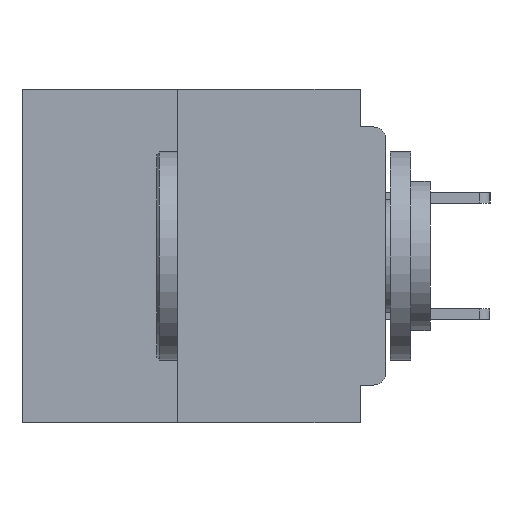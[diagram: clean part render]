
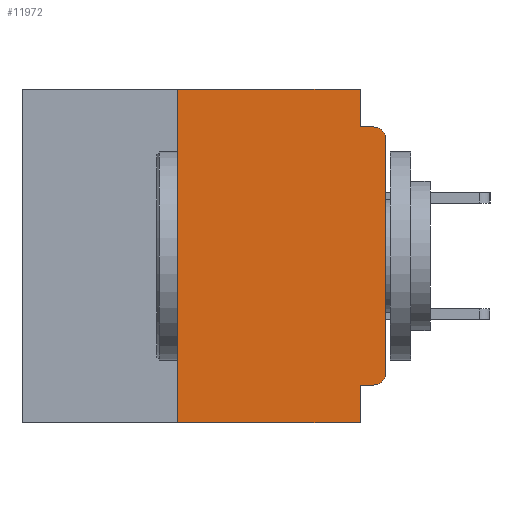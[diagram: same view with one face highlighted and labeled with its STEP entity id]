
A CAD part, left-side view. The second image highlights one B-rep face of the part: STEP entity #11972.
In plain terms, the highlighted planar face has unit normal (-1, 0, 0).
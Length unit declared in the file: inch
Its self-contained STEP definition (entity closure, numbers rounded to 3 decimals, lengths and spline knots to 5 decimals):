
#702 = VERTEX_POINT ( 'NONE', #54843 ) ;
#1811 = VERTEX_POINT ( 'NONE', #20018 ) ;
#4712 = CARTESIAN_POINT ( 'NONE',  ( 0., 0.437, 0. ) ) ;
#7472 = CARTESIAN_POINT ( 'NONE',  ( 0., 0.437, -0.4 ) ) ;
#7946 = EDGE_CURVE ( 'NONE', #57414, #702, #52323, .T. ) ;
#8052 = CARTESIAN_POINT ( 'NONE',  ( 0., 0.031, -0.355 ) ) ;
#8495 = CARTESIAN_POINT ( 'NONE',  ( 0., 0.031, 0. ) ) ;
#9352 = CARTESIAN_POINT ( 'NONE',  ( 0., 0.031, -0.4 ) ) ;
#9737 = VECTOR ( 'NONE', #40722, 39.37008 ) ;
#9796 = DIRECTION ( 'NONE',  ( 0., 1., 0. ) ) ;
#10257 = VERTEX_POINT ( 'NONE', #26224 ) ;
#11354 = LINE ( 'NONE', #14819, #9737 ) ;
#11581 = VECTOR ( 'NONE', #56571, 39.37008 ) ;
#11972 = ADVANCED_FACE ( 'NONE', ( #33590 ), #56384, .F. ) ;
#12123 = CARTESIAN_POINT ( 'NONE',  ( 0., 0.25, 0. ) ) ;
#12883 = CARTESIAN_POINT ( 'NONE',  ( 0., 0.25, -0.4 ) ) ;
#13682 = DIRECTION ( 'NONE',  ( 0., 0., -1. ) ) ;
#14777 = CARTESIAN_POINT ( 'NONE',  ( 0., 0., -0.355 ) ) ;
#14819 = CARTESIAN_POINT ( 'NONE',  ( 0., 0.437, 0. ) ) ;
#15334 = VECTOR ( 'NONE', #64381, 39.37008 ) ;
#15539 = EDGE_CURVE ( 'NONE', #24366, #20336, #37382, .T. ) ;
#15829 = VERTEX_POINT ( 'NONE', #12123 ) ;
#15956 = EDGE_CURVE ( 'NONE', #702, #58829, #66434, .T. ) ;
#17506 = ORIENTED_EDGE ( 'NONE', *, *, #32362, .T. ) ;
#18109 = DIRECTION ( 'NONE',  ( 0., 0., 1. ) ) ;
#18802 = VECTOR ( 'NONE', #18109, 39.37008 ) ;
#20018 = CARTESIAN_POINT ( 'NONE',  ( 0., 0.015, -0.355 ) ) ;
#20336 = VERTEX_POINT ( 'NONE', #33363 ) ;
#20462 = AXIS2_PLACEMENT_3D ( 'NONE', #58294, #27416, #63546 ) ;
#20517 = CARTESIAN_POINT ( 'NONE',  ( 0., 0., 0. ) ) ;
#20711 = ORIENTED_EDGE ( 'NONE', *, *, #48529, .F. ) ;
#21270 = VERTEX_POINT ( 'NONE', #9352 ) ;
#23662 = VECTOR ( 'NONE', #55121, 39.37008 ) ;
#24366 = VERTEX_POINT ( 'NONE', #45286 ) ;
#24946 = VECTOR ( 'NONE', #13682, 39.37008 ) ;
#25868 = DIRECTION ( 'NONE',  ( 0., 0., -1. ) ) ;
#26224 = CARTESIAN_POINT ( 'NONE',  ( 0., 0.25, -0.4 ) ) ;
#27063 = LINE ( 'NONE', #14777, #39095 ) ;
#27416 = DIRECTION ( 'NONE',  ( -1., 0., 0. ) ) ;
#27942 = ORIENTED_EDGE ( 'NONE', *, *, #15539, .T. ) ;
#28408 = EDGE_LOOP ( 'NONE', ( #27942, #17506, #58764, #44585, #45764, #40111, #41410, #20711, #46842, #46403 ) ) ;
#30639 = DIRECTION ( 'NONE',  ( -1., 0., 0. ) ) ;
#30701 = DIRECTION ( 'NONE',  ( 0., 0., -1. ) ) ;
#30741 = VECTOR ( 'NONE', #25868, 39.37008 ) ;
#32362 = EDGE_CURVE ( 'NONE', #20336, #58829, #54423, .T. ) ;
#33363 = CARTESIAN_POINT ( 'NONE',  ( 0., 0., -0.06 ) ) ;
#33590 = FACE_OUTER_BOUND ( 'NONE', #28408, .T. ) ;
#34231 = CIRCLE ( 'NONE', #20462, 0.015 ) ;
#37382 = LINE ( 'NONE', #20517, #11581 ) ;
#37975 = EDGE_CURVE ( 'NONE', #10257, #15829, #44560, .T. ) ;
#38454 = CARTESIAN_POINT ( 'NONE',  ( 0., 0.031, 0. ) ) ;
#39095 = VECTOR ( 'NONE', #9796, 39.37008 ) ;
#40111 = ORIENTED_EDGE ( 'NONE', *, *, #37975, .F. ) ;
#40722 = DIRECTION ( 'NONE',  ( 0., -1., 0. ) ) ;
#40737 = EDGE_CURVE ( 'NONE', #10257, #21270, #56467, .T. ) ;
#41410 = ORIENTED_EDGE ( 'NONE', *, *, #40737, .T. ) ;
#41702 = AXIS2_PLACEMENT_3D ( 'NONE', #4712, #61636, #30701 ) ;
#44442 = LINE ( 'NONE', #56715, #30741 ) ;
#44560 = LINE ( 'NONE', #12883, #18802 ) ;
#44579 = VERTEX_POINT ( 'NONE', #8052 ) ;
#44585 = ORIENTED_EDGE ( 'NONE', *, *, #7946, .F. ) ;
#45286 = CARTESIAN_POINT ( 'NONE',  ( 0., 0., -0.34 ) ) ;
#45764 = ORIENTED_EDGE ( 'NONE', *, *, #54713, .F. ) ;
#46403 = ORIENTED_EDGE ( 'NONE', *, *, #52588, .T. ) ;
#46842 = ORIENTED_EDGE ( 'NONE', *, *, #57698, .F. ) ;
#48529 = EDGE_CURVE ( 'NONE', #44579, #21270, #44442, .T. ) ;
#50000 = CARTESIAN_POINT ( 'NONE',  ( 0., 0.015, -0.045 ) ) ;
#52323 = LINE ( 'NONE', #8495, #24946 ) ;
#52588 = EDGE_CURVE ( 'NONE', #1811, #24366, #34231, .T. ) ;
#54423 = CIRCLE ( 'NONE', #61899, 0.015 ) ;
#54713 = EDGE_CURVE ( 'NONE', #15829, #57414, #11354, .T. ) ;
#54843 = CARTESIAN_POINT ( 'NONE',  ( 0., 0.031, -0.045 ) ) ;
#55121 = DIRECTION ( 'NONE',  ( 0., -1., 0. ) ) ;
#56384 = PLANE ( 'NONE',  #41702 ) ;
#56467 = LINE ( 'NONE', #7472, #15334 ) ;
#56571 = DIRECTION ( 'NONE',  ( 0., 0., 1. ) ) ;
#56715 = CARTESIAN_POINT ( 'NONE',  ( 0., 0.031, -0.4 ) ) ;
#57414 = VERTEX_POINT ( 'NONE', #38454 ) ;
#57698 = EDGE_CURVE ( 'NONE', #1811, #44579, #27063, .T. ) ;
#58294 = CARTESIAN_POINT ( 'NONE',  ( 0., 0.015, -0.34 ) ) ;
#58764 = ORIENTED_EDGE ( 'NONE', *, *, #15956, .F. ) ;
#58829 = VERTEX_POINT ( 'NONE', #50000 ) ;
#60363 = CARTESIAN_POINT ( 'NONE',  ( 0., 0., -0.045 ) ) ;
#61565 = CARTESIAN_POINT ( 'NONE',  ( 0., 0.015, -0.06 ) ) ;
#61636 = DIRECTION ( 'NONE',  ( 1., 0., 0. ) ) ;
#61899 = AXIS2_PLACEMENT_3D ( 'NONE', #61565, #30639, #66747 ) ;
#63546 = DIRECTION ( 'NONE',  ( 0., 0., -1. ) ) ;
#64381 = DIRECTION ( 'NONE',  ( 0., -1., 0. ) ) ;
#66434 = LINE ( 'NONE', #60363, #23662 ) ;
#66747 = DIRECTION ( 'NONE',  ( 0., 0., -1. ) ) ;
